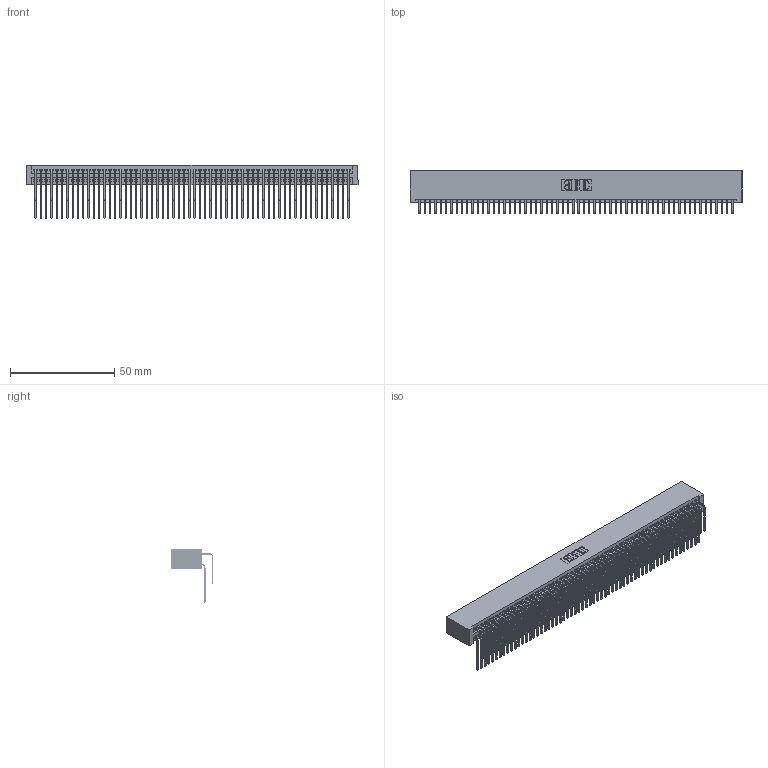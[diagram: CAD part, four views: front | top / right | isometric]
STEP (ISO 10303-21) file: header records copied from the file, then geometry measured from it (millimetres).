
FILE_DESCRIPTION (( 'STEP AP203' ), '1' );
FILE_NAME ('345-120-559-201.STEP', '2019-11-06T04:19:37', ( '' ), ( '' ), 'SwSTEP 2.0', 'SolidWorks 2016', '' );
FILE_SCHEMA (( 'CONFIG_CONTROL_DESIGN' ));
Length unit declared in the file: inch
Products named in the file (4): 345-292-001_559 Tail - 2; 345-120-559-201; 345 Part_No Mounting Lugs; 345-292-001_558 559 Tail - 1
Assembly tree (121 placements, depth 2):
  345-120-559-201
    345 Part_No Mounting Lugs
    345-292-001_558 559 Tail - 1  x60
    345-292-001_559 Tail - 2  x60
Bounding box: 159 x 20.56 x 25.53 mm (x, y, z)
Volume: 16921 mm3; surface area: 28919.2 mm2
Topology: 121 solids, 121 shells, 6358 faces, 18917 edges, 12450 vertices
Faces by surface type: plane 4276, cylinder 2082
Entity records: 46029 total; most frequent: CARTESIAN_POINT 7743, ORIENTED_EDGE 7626, DIRECTION 6773, EDGE_CURVE 3813, LINE 3409, VECTOR 3409, VERTEX_POINT 2538, AXIS2_PLACEMENT_3D 1682
